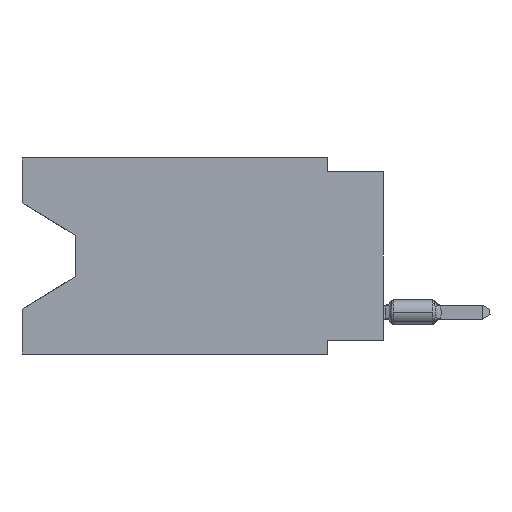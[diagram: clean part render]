
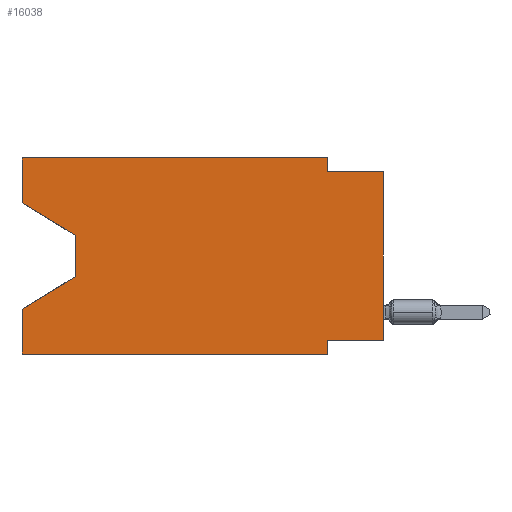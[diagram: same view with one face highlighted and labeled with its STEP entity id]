
A CAD part, left-side view. The second image highlights one B-rep face of the part: STEP entity #16038.
In plain terms, the highlighted planar face has unit normal (-1, 0, 0).
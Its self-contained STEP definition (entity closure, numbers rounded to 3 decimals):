
#5 = ORIENTED_EDGE ( 'NONE', *, *, #23384, .T. ) ;
#623 = VECTOR ( 'NONE', #1859, 1000. ) ;
#660 = VECTOR ( 'NONE', #20025, 1000. ) ;
#950 = LINE ( 'NONE', #36917, #33658 ) ;
#1053 = LINE ( 'NONE', #32735, #10181 ) ;
#1151 = VERTEX_POINT ( 'NONE', #9040 ) ;
#1770 = CARTESIAN_POINT ( 'NONE',  ( 0., 13.97, -3.505 ) ) ;
#1804 = DIRECTION ( 'NONE',  ( 0., 1., 0. ) ) ;
#1859 = DIRECTION ( 'NONE',  ( 0., -1., 0. ) ) ;
#1971 = EDGE_CURVE ( 'NONE', #12186, #25576, #34052, .T. ) ;
#2057 = LINE ( 'NONE', #31889, #660 ) ;
#2538 = DIRECTION ( 'NONE',  ( 0., 0., 1. ) ) ;
#3013 = CARTESIAN_POINT ( 'NONE',  ( 0., 2.54, 0. ) ) ;
#3178 = VERTEX_POINT ( 'NONE', #23888 ) ;
#3415 = ORIENTED_EDGE ( 'NONE', *, *, #30512, .T. ) ;
#3845 = VECTOR ( 'NONE', #13457, 1000. ) ;
#4043 = DIRECTION ( 'NONE',  ( 0., -1., 0. ) ) ;
#4146 = VERTEX_POINT ( 'NONE', #19752 ) ;
#6792 = DIRECTION ( 'NONE',  ( 0., 0., -1. ) ) ;
#8493 = ORIENTED_EDGE ( 'NONE', *, *, #13706, .T. ) ;
#8615 = VERTEX_POINT ( 'NONE', #22520 ) ;
#9040 = CARTESIAN_POINT ( 'NONE',  ( 0., 2.54, -0.635 ) ) ;
#9474 = VECTOR ( 'NONE', #21212, 1000. ) ;
#10008 = CARTESIAN_POINT ( 'NONE',  ( 0., 0., -0.635 ) ) ;
#10079 = EDGE_CURVE ( 'NONE', #4146, #35447, #31420, .T. ) ;
#10181 = VECTOR ( 'NONE', #6792, 1000. ) ;
#10380 = EDGE_CURVE ( 'NONE', #3178, #13452, #16822, .T. ) ;
#11098 = DIRECTION ( 'NONE',  ( 0., -1., 0. ) ) ;
#11184 = EDGE_CURVE ( 'NONE', #25576, #1151, #1053, .T. ) ;
#11338 = ORIENTED_EDGE ( 'NONE', *, *, #29813, .F. ) ;
#11479 = AXIS2_PLACEMENT_3D ( 'NONE', #24604, #13149, #25197 ) ;
#11820 = DIRECTION ( 'NONE',  ( 0., 0., 1. ) ) ;
#12186 = VERTEX_POINT ( 'NONE', #14575 ) ;
#12373 = PLANE ( 'NONE',  #11479 ) ;
#12950 = EDGE_CURVE ( 'NONE', #24165, #12186, #950, .T. ) ;
#12956 = FACE_OUTER_BOUND ( 'NONE', #28768, .T. ) ;
#13149 = DIRECTION ( 'NONE',  ( 1., 0., 0. ) ) ;
#13296 = CARTESIAN_POINT ( 'NONE',  ( 0., 0., -8.255 ) ) ;
#13452 = VERTEX_POINT ( 'NONE', #34286 ) ;
#13457 = DIRECTION ( 'NONE',  ( 0., 0., -1. ) ) ;
#13463 = EDGE_CURVE ( 'NONE', #1151, #8615, #25979, .T. ) ;
#13706 = EDGE_CURVE ( 'NONE', #35447, #29016, #24173, .T. ) ;
#14366 = EDGE_CURVE ( 'NONE', #24165, #4146, #2057, .T. ) ;
#14575 = CARTESIAN_POINT ( 'NONE',  ( 0., 16.383, 0. ) ) ;
#14647 = CARTESIAN_POINT ( 'NONE',  ( 0., 16.383, -8.89 ) ) ;
#16038 = ADVANCED_FACE ( 'NONE', ( #12956 ), #12373, .F. ) ;
#16257 = CARTESIAN_POINT ( 'NONE',  ( 0., 16.383, -2.038 ) ) ;
#16822 = LINE ( 'NONE', #13296, #34795 ) ;
#17833 = DIRECTION ( 'NONE',  ( 0., 0., -1. ) ) ;
#19665 = ORIENTED_EDGE ( 'NONE', *, *, #10079, .T. ) ;
#19752 = CARTESIAN_POINT ( 'NONE',  ( 0., 13.97, -3.505 ) ) ;
#19842 = CARTESIAN_POINT ( 'NONE',  ( 0., 13.97, -5.385 ) ) ;
#20025 = DIRECTION ( 'NONE',  ( 0., -0.855, -0.519 ) ) ;
#20741 = ORIENTED_EDGE ( 'NONE', *, *, #12950, .F. ) ;
#20932 = EDGE_CURVE ( 'NONE', #13452, #26692, #32852, .T. ) ;
#21212 = DIRECTION ( 'NONE',  ( 0., 0.855, -0.519 ) ) ;
#22287 = ORIENTED_EDGE ( 'NONE', *, *, #10380, .F. ) ;
#22520 = CARTESIAN_POINT ( 'NONE',  ( 0., 0., -0.635 ) ) ;
#23384 = EDGE_CURVE ( 'NONE', #3178, #8615, #29605, .T. ) ;
#23864 = ORIENTED_EDGE ( 'NONE', *, *, #20932, .F. ) ;
#23888 = CARTESIAN_POINT ( 'NONE',  ( 0., 0., -8.255 ) ) ;
#24165 = VERTEX_POINT ( 'NONE', #16257 ) ;
#24173 = LINE ( 'NONE', #33852, #9474 ) ;
#24604 = CARTESIAN_POINT ( 'NONE',  ( 0., 16.383, 0. ) ) ;
#25197 = DIRECTION ( 'NONE',  ( 0., 0., -1. ) ) ;
#25514 = CARTESIAN_POINT ( 'NONE',  ( 0., 16.383, -6.852 ) ) ;
#25576 = VERTEX_POINT ( 'NONE', #3013 ) ;
#25979 = LINE ( 'NONE', #10008, #623 ) ;
#26106 = LINE ( 'NONE', #38161, #36155 ) ;
#26692 = VERTEX_POINT ( 'NONE', #28935 ) ;
#26836 = CARTESIAN_POINT ( 'NONE',  ( 0., 16.383, 0. ) ) ;
#27033 = CARTESIAN_POINT ( 'NONE',  ( 0., 0., 0. ) ) ;
#27505 = VECTOR ( 'NONE', #4043, 1000. ) ;
#28034 = DIRECTION ( 'NONE',  ( 0., 0., 1. ) ) ;
#28526 = CARTESIAN_POINT ( 'NONE',  ( 0., 16.383, 0. ) ) ;
#28768 = EDGE_LOOP ( 'NONE', ( #37685, #19665, #8493, #11338, #3415, #23864, #22287, #5, #31078, #33542, #38537, #20741 ) ) ;
#28935 = CARTESIAN_POINT ( 'NONE',  ( 0., 2.54, -8.89 ) ) ;
#29016 = VERTEX_POINT ( 'NONE', #25514 ) ;
#29605 = LINE ( 'NONE', #27033, #37631 ) ;
#29813 = EDGE_CURVE ( 'NONE', #33805, #29016, #32757, .T. ) ;
#30271 = CARTESIAN_POINT ( 'NONE',  ( 0., 2.54, -8.89 ) ) ;
#30512 = EDGE_CURVE ( 'NONE', #33805, #26692, #26106, .T. ) ;
#31078 = ORIENTED_EDGE ( 'NONE', *, *, #13463, .F. ) ;
#31420 = LINE ( 'NONE', #1770, #3845 ) ;
#31889 = CARTESIAN_POINT ( 'NONE',  ( 0., 16.383, -2.038 ) ) ;
#32735 = CARTESIAN_POINT ( 'NONE',  ( 0., 2.54, 0. ) ) ;
#32757 = LINE ( 'NONE', #26836, #34536 ) ;
#32852 = LINE ( 'NONE', #30271, #38102 ) ;
#33542 = ORIENTED_EDGE ( 'NONE', *, *, #11184, .F. ) ;
#33658 = VECTOR ( 'NONE', #28034, 1000. ) ;
#33805 = VERTEX_POINT ( 'NONE', #14647 ) ;
#33852 = CARTESIAN_POINT ( 'NONE',  ( 0., 13.97, -5.385 ) ) ;
#34052 = LINE ( 'NONE', #28526, #27505 ) ;
#34286 = CARTESIAN_POINT ( 'NONE',  ( 0., 2.54, -8.255 ) ) ;
#34536 = VECTOR ( 'NONE', #11820, 1000. ) ;
#34795 = VECTOR ( 'NONE', #1804, 1000. ) ;
#35447 = VERTEX_POINT ( 'NONE', #19842 ) ;
#36155 = VECTOR ( 'NONE', #11098, 1000. ) ;
#36917 = CARTESIAN_POINT ( 'NONE',  ( 0., 16.383, 0. ) ) ;
#37631 = VECTOR ( 'NONE', #2538, 1000. ) ;
#37685 = ORIENTED_EDGE ( 'NONE', *, *, #14366, .T. ) ;
#38102 = VECTOR ( 'NONE', #17833, 1000. ) ;
#38161 = CARTESIAN_POINT ( 'NONE',  ( 0., 16.383, -8.89 ) ) ;
#38537 = ORIENTED_EDGE ( 'NONE', *, *, #1971, .F. ) ;
